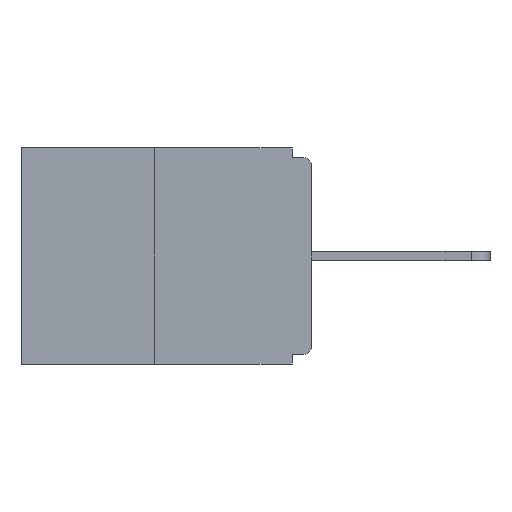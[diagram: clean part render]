
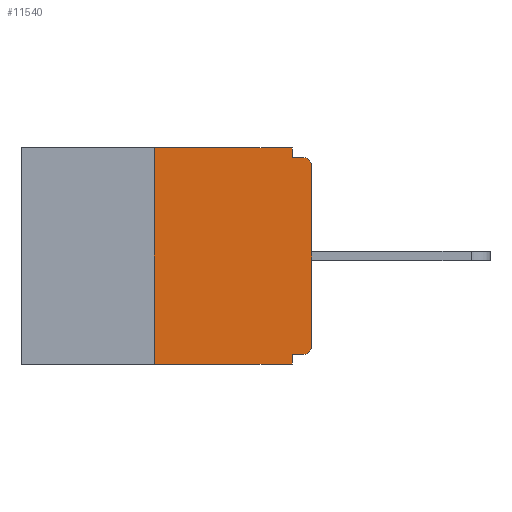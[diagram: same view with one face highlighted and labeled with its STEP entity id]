
A CAD part, left-side view. The second image highlights one B-rep face of the part: STEP entity #11540.
In plain terms, the highlighted planar face has unit normal (-1, 0, 0).
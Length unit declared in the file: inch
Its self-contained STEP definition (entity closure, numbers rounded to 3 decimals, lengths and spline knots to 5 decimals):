
#447 = ORIENTED_EDGE ( 'NONE', *, *, #18250, .T. ) ;
#549 = VECTOR ( 'NONE', #11100, 39.37008 ) ;
#971 = DIRECTION ( 'NONE',  ( 0., 0., -1. ) ) ;
#1357 = VECTOR ( 'NONE', #16246, 39.37008 ) ;
#1376 = LINE ( 'NONE', #13928, #14189 ) ;
#1973 = CARTESIAN_POINT ( 'NONE',  ( 0., 0.46, 0. ) ) ;
#2084 = CARTESIAN_POINT ( 'NONE',  ( 0., 0.031, -0.343 ) ) ;
#2172 = DIRECTION ( 'NONE',  ( 1., 0., 0. ) ) ;
#2285 = CARTESIAN_POINT ( 'NONE',  ( 0., 0.031, -0.328 ) ) ;
#2450 = ORIENTED_EDGE ( 'NONE', *, *, #9689, .T. ) ;
#2690 = ORIENTED_EDGE ( 'NONE', *, *, #6247, .F. ) ;
#3187 = CARTESIAN_POINT ( 'NONE',  ( 0., 0., 0. ) ) ;
#3478 = LINE ( 'NONE', #16143, #549 ) ;
#3479 = VECTOR ( 'NONE', #12369, 39.37008 ) ;
#3607 = ORIENTED_EDGE ( 'NONE', *, *, #8856, .T. ) ;
#4072 = CARTESIAN_POINT ( 'NONE',  ( 0., 0.031, -0.343 ) ) ;
#4121 = ORIENTED_EDGE ( 'NONE', *, *, #8039, .F. ) ;
#4512 = CARTESIAN_POINT ( 'NONE',  ( 0., 0.25, 0. ) ) ;
#4708 = VERTEX_POINT ( 'NONE', #17601 ) ;
#4892 = LINE ( 'NONE', #3187, #6499 ) ;
#5622 = EDGE_CURVE ( 'NONE', #16680, #4708, #1376, .T. ) ;
#5798 = EDGE_CURVE ( 'NONE', #20200, #11868, #5868, .T. ) ;
#5868 = LINE ( 'NONE', #11432, #1357 ) ;
#6114 = VERTEX_POINT ( 'NONE', #4072 ) ;
#6247 = EDGE_CURVE ( 'NONE', #4708, #8116, #3478, .T. ) ;
#6499 = VECTOR ( 'NONE', #6780, 39.37008 ) ;
#6780 = DIRECTION ( 'NONE',  ( 0., 0., 1. ) ) ;
#6871 = DIRECTION ( 'NONE',  ( 0., 0., -1. ) ) ;
#7408 = CIRCLE ( 'NONE', #7516, 0.015 ) ;
#7516 = AXIS2_PLACEMENT_3D ( 'NONE', #8650, #17054, #6871 ) ;
#7945 = EDGE_CURVE ( 'NONE', #20200, #10202, #15994, .T. ) ;
#8039 = EDGE_CURVE ( 'NONE', #11868, #6114, #13092, .T. ) ;
#8116 = VERTEX_POINT ( 'NONE', #11158 ) ;
#8154 = DIRECTION ( 'NONE',  ( 0., -1., 0. ) ) ;
#8172 = FACE_OUTER_BOUND ( 'NONE', #17264, .T. ) ;
#8650 = CARTESIAN_POINT ( 'NONE',  ( 0., 0.015, -0.03 ) ) ;
#8717 = VERTEX_POINT ( 'NONE', #9993 ) ;
#8856 = EDGE_CURVE ( 'NONE', #8717, #6114, #9286, .T. ) ;
#9286 = LINE ( 'NONE', #16868, #21021 ) ;
#9689 = EDGE_CURVE ( 'NONE', #19441, #8116, #7408, .T. ) ;
#9704 = CARTESIAN_POINT ( 'NONE',  ( 0., 0.015, -0.313 ) ) ;
#9843 = VECTOR ( 'NONE', #12784, 39.37008 ) ;
#9993 = CARTESIAN_POINT ( 'NONE',  ( 0., 0.25, -0.343 ) ) ;
#10068 = VERTEX_POINT ( 'NONE', #4512 ) ;
#10202 = VERTEX_POINT ( 'NONE', #15445 ) ;
#10492 = VECTOR ( 'NONE', #8154, 39.37008 ) ;
#10714 = EDGE_CURVE ( 'NONE', #8717, #10068, #12209, .T. ) ;
#11100 = DIRECTION ( 'NONE',  ( 0., -1., 0. ) ) ;
#11158 = CARTESIAN_POINT ( 'NONE',  ( 0., 0.015, -0.015 ) ) ;
#11340 = ORIENTED_EDGE ( 'NONE', *, *, #10714, .F. ) ;
#11432 = CARTESIAN_POINT ( 'NONE',  ( 0., 0., -0.328 ) ) ;
#11540 = ADVANCED_FACE ( 'NONE', ( #8172 ), #19083, .F. ) ;
#11868 = VERTEX_POINT ( 'NONE', #2285 ) ;
#12190 = ORIENTED_EDGE ( 'NONE', *, *, #15995, .F. ) ;
#12209 = LINE ( 'NONE', #14566, #9843 ) ;
#12369 = DIRECTION ( 'NONE',  ( 0., 0., -1. ) ) ;
#12784 = DIRECTION ( 'NONE',  ( 0., 0., 1. ) ) ;
#13092 = LINE ( 'NONE', #2084, #3479 ) ;
#13143 = DIRECTION ( 'NONE',  ( -1., 0., 0. ) ) ;
#13555 = ORIENTED_EDGE ( 'NONE', *, *, #5798, .F. ) ;
#13603 = CARTESIAN_POINT ( 'NONE',  ( 0., 0., -0.03 ) ) ;
#13906 = DIRECTION ( 'NONE',  ( 0., 0., -1. ) ) ;
#13928 = CARTESIAN_POINT ( 'NONE',  ( 0., 0.031, 0. ) ) ;
#14189 = VECTOR ( 'NONE', #15610, 39.37008 ) ;
#14566 = CARTESIAN_POINT ( 'NONE',  ( 0., 0.25, 0. ) ) ;
#15445 = CARTESIAN_POINT ( 'NONE',  ( 0., 0., -0.313 ) ) ;
#15610 = DIRECTION ( 'NONE',  ( 0., 0., -1. ) ) ;
#15868 = AXIS2_PLACEMENT_3D ( 'NONE', #9704, #13143, #971 ) ;
#15994 = CIRCLE ( 'NONE', #15868, 0.015 ) ;
#15995 = EDGE_CURVE ( 'NONE', #10068, #16680, #20065, .T. ) ;
#16143 = CARTESIAN_POINT ( 'NONE',  ( 0., 0., -0.015 ) ) ;
#16246 = DIRECTION ( 'NONE',  ( 0., 1., 0. ) ) ;
#16680 = VERTEX_POINT ( 'NONE', #18991 ) ;
#16868 = CARTESIAN_POINT ( 'NONE',  ( 0., 0.46, -0.343 ) ) ;
#17054 = DIRECTION ( 'NONE',  ( -1., 0., 0. ) ) ;
#17264 = EDGE_LOOP ( 'NONE', ( #12190, #11340, #3607, #4121, #13555, #18902, #447, #2450, #2690, #19192 ) ) ;
#17601 = CARTESIAN_POINT ( 'NONE',  ( 0., 0.031, -0.015 ) ) ;
#18204 = AXIS2_PLACEMENT_3D ( 'NONE', #1973, #2172, #13906 ) ;
#18250 = EDGE_CURVE ( 'NONE', #10202, #19441, #4892, .T. ) ;
#18340 = CARTESIAN_POINT ( 'NONE',  ( 0., 0.46, 0. ) ) ;
#18503 = DIRECTION ( 'NONE',  ( 0., -1., 0. ) ) ;
#18902 = ORIENTED_EDGE ( 'NONE', *, *, #7945, .T. ) ;
#18991 = CARTESIAN_POINT ( 'NONE',  ( 0., 0.031, 0. ) ) ;
#19083 = PLANE ( 'NONE',  #18204 ) ;
#19124 = CARTESIAN_POINT ( 'NONE',  ( 0., 0.015, -0.328 ) ) ;
#19192 = ORIENTED_EDGE ( 'NONE', *, *, #5622, .F. ) ;
#19441 = VERTEX_POINT ( 'NONE', #13603 ) ;
#20065 = LINE ( 'NONE', #18340, #10492 ) ;
#20200 = VERTEX_POINT ( 'NONE', #19124 ) ;
#21021 = VECTOR ( 'NONE', #18503, 39.37008 ) ;
